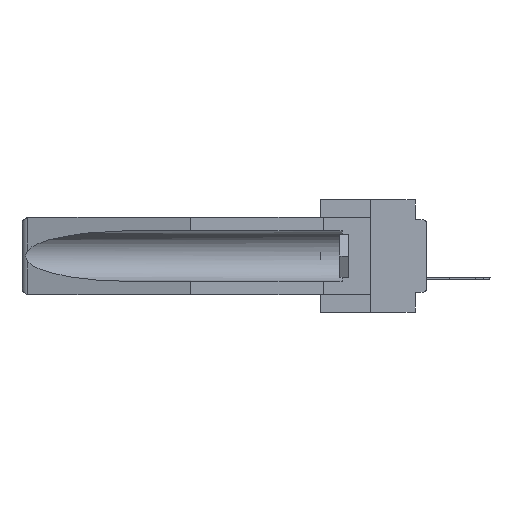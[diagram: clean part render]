
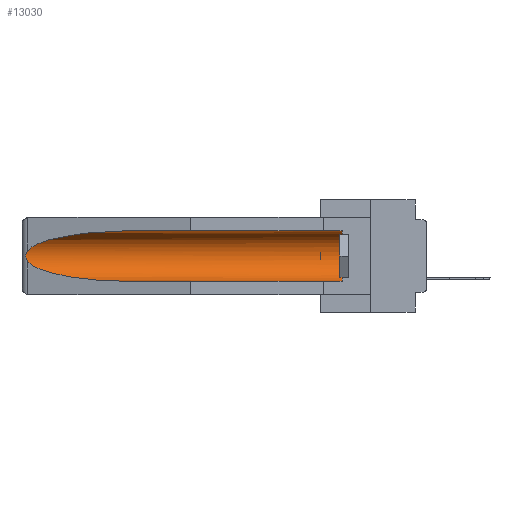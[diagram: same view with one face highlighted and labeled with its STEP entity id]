
A CAD part, left-side view. The second image highlights one B-rep face of the part: STEP entity #13030.
In plain terms, the highlighted cylindrical face has radius 2.857 mm (diameter 5.715 mm), a partial arc.
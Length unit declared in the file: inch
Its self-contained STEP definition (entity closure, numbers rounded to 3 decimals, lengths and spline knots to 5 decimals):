
#1356 = CARTESIAN_POINT ( 'NONE',  ( 0.26597, 1.5296, -0.19026 ) ) ;
#1966 = AXIS2_PLACEMENT_3D ( 'NONE', #36388, #32983, #39023 ) ;
#2346 = CARTESIAN_POINT ( 'NONE',  ( 0.26537, 1.52718, -0.19328 ) ) ;
#2478 = CARTESIAN_POINT ( 'NONE',  ( 0.155, 1.07973, -0.284 ) ) ;
#2673 = DIRECTION ( 'NONE',  ( 0., 1., 0. ) ) ;
#2771 = ORIENTED_EDGE ( 'NONE', *, *, #6622, .T. ) ;
#2885 = B_SPLINE_CURVE_WITH_KNOTS ( 'NONE', 3,
 ( #12368, #5298, #27321, #39610, #24892, #18644, #30938, #13312, #1356, #13907 ),
 .UNSPECIFIED., .F., .F.,
 ( 4, 2, 2, 2, 4 ),
 ( 0., 0.00029, 0.00058, 0.00087, 0.00117 ),
 .UNSPECIFIED. ) ;
#3277 = LINE ( 'NONE', #30534, #9221 ) ;
#4219 = VECTOR ( 'NONE', #39532, 39.37008 ) ;
#4569 = CIRCLE ( 'NONE', #1966, 0.1125 ) ;
#4816 = DIRECTION ( 'NONE',  ( 0., 0., 1. ) ) ;
#5298 = CARTESIAN_POINT ( 'NONE',  ( 0.26597, 1.52961, -0.15275 ) ) ;
#5886 = CARTESIAN_POINT ( 'NONE',  ( 0.26537, 1.52718, -0.14972 ) ) ;
#6622 = EDGE_CURVE ( 'NONE', #8143, #30828, #2885, .T. ) ;
#6766 = CARTESIAN_POINT ( 'NONE',  ( 0.26537, 1.52718, -0.14972 ) ) ;
#7658 = EDGE_CURVE ( 'NONE', #30828, #13727, #8458, .T. ) ;
#8143 = VERTEX_POINT ( 'NONE', #5886 ) ;
#8458 =( BOUNDED_CURVE ( )  B_SPLINE_CURVE ( 3, ( #2346, #13892, #14704, #26816 ),
 .UNSPECIFIED., .F., .F. ) 
 B_SPLINE_CURVE_WITH_KNOTS ( ( 4, 4 ),
 ( 0.1948, 1.5708 ),
 .UNSPECIFIED. ) 
 CURVE ( )  GEOMETRIC_REPRESENTATION_ITEM ( )  RATIONAL_B_SPLINE_CURVE ( ( 1., 0.848, 0.848, 1. ) ) 
 REPRESENTATION_ITEM ( '' )  );
#9221 = VECTOR ( 'NONE', #2673, 39.37008 ) ;
#9334 = EDGE_LOOP ( 'NONE', ( #15441, #2771, #26582, #38266, #13902, #19964 ) ) ;
#10158 = EDGE_CURVE ( 'NONE', #10968, #8143, #21922, .T. ) ;
#10476 = CYLINDRICAL_SURFACE ( 'NONE', #32827, 0.1125 ) ;
#10968 = VERTEX_POINT ( 'NONE', #15533 ) ;
#11083 = CARTESIAN_POINT ( 'NONE',  ( 0.155, -0.30754, -0.1715 ) ) ;
#12368 = CARTESIAN_POINT ( 'NONE',  ( 0.26537, 1.52718, -0.14972 ) ) ;
#13030 = ADVANCED_FACE ( 'NONE', ( #13712 ), #10476, .F. ) ;
#13312 = CARTESIAN_POINT ( 'NONE',  ( 0.26655, 1.53094, -0.18657 ) ) ;
#13712 = FACE_OUTER_BOUND ( 'NONE', #9334, .T. ) ;
#13727 = VERTEX_POINT ( 'NONE', #2478 ) ;
#13809 = CARTESIAN_POINT ( 'NONE',  ( 0.155, 0.126, -0.059 ) ) ;
#13892 = CARTESIAN_POINT ( 'NONE',  ( 0.25451, 1.48313, -0.24835 ) ) ;
#13902 = ORIENTED_EDGE ( 'NONE', *, *, #17924, .T. ) ;
#13907 = CARTESIAN_POINT ( 'NONE',  ( 0.26537, 1.52718, -0.19328 ) ) ;
#14704 = CARTESIAN_POINT ( 'NONE',  ( 0.21114, 1.30732, -0.284 ) ) ;
#15441 = ORIENTED_EDGE ( 'NONE', *, *, #10158, .T. ) ;
#15533 = CARTESIAN_POINT ( 'NONE',  ( 0.155, 1.07973, -0.059 ) ) ;
#17759 = CARTESIAN_POINT ( 'NONE',  ( 0.155, -0.30754, -0.284 ) ) ;
#17924 = EDGE_CURVE ( 'NONE', #27974, #25676, #4569, .T. ) ;
#18644 = CARTESIAN_POINT ( 'NONE',  ( 0.2675, 1.53308, -0.17534 ) ) ;
#18715 = CARTESIAN_POINT ( 'NONE',  ( 0.21114, 1.30732, -0.059 ) ) ;
#19964 = ORIENTED_EDGE ( 'NONE', *, *, #23916, .T. ) ;
#21922 =( BOUNDED_CURVE ( )  B_SPLINE_CURVE ( 3, ( #34418, #18715, #31002, #6766 ),
 .UNSPECIFIED., .F., .T. ) 
 B_SPLINE_CURVE_WITH_KNOTS ( ( 4, 4 ),
 ( 4.71239, 6.08839 ),
 .UNSPECIFIED. ) 
 CURVE ( )  GEOMETRIC_REPRESENTATION_ITEM ( )  RATIONAL_B_SPLINE_CURVE ( ( 1., 0.848, 0.848, 1. ) ) 
 REPRESENTATION_ITEM ( '' )  );
#22816 = DIRECTION ( 'NONE',  ( 0., 1., 0. ) ) ;
#23916 = EDGE_CURVE ( 'NONE', #25676, #10968, #3277, .T. ) ;
#24892 = CARTESIAN_POINT ( 'NONE',  ( 0.2675, 1.53308, -0.16763 ) ) ;
#25676 = VERTEX_POINT ( 'NONE', #13809 ) ;
#26582 = ORIENTED_EDGE ( 'NONE', *, *, #7658, .T. ) ;
#26816 = CARTESIAN_POINT ( 'NONE',  ( 0.155, 1.07973, -0.284 ) ) ;
#27321 = CARTESIAN_POINT ( 'NONE',  ( 0.26654, 1.53092, -0.15636 ) ) ;
#27974 = VERTEX_POINT ( 'NONE', #36399 ) ;
#30534 = CARTESIAN_POINT ( 'NONE',  ( 0.155, -0.30754, -0.059 ) ) ;
#30828 = VERTEX_POINT ( 'NONE', #38042 ) ;
#30938 = CARTESIAN_POINT ( 'NONE',  ( 0.2673, 1.53269, -0.17917 ) ) ;
#31002 = CARTESIAN_POINT ( 'NONE',  ( 0.25451, 1.48313, -0.09465 ) ) ;
#32827 = AXIS2_PLACEMENT_3D ( 'NONE', #11083, #22816, #4816 ) ;
#32983 = DIRECTION ( 'NONE',  ( 0., -1., 0. ) ) ;
#33095 = LINE ( 'NONE', #17759, #4219 ) ;
#34418 = CARTESIAN_POINT ( 'NONE',  ( 0.155, 1.07973, -0.059 ) ) ;
#36388 = CARTESIAN_POINT ( 'NONE',  ( 0.155, 0.126, -0.1715 ) ) ;
#36399 = CARTESIAN_POINT ( 'NONE',  ( 0.155, 0.126, -0.284 ) ) ;
#36586 = EDGE_CURVE ( 'NONE', #27974, #13727, #33095, .T. ) ;
#38042 = CARTESIAN_POINT ( 'NONE',  ( 0.26537, 1.52718, -0.19328 ) ) ;
#38266 = ORIENTED_EDGE ( 'NONE', *, *, #36586, .F. ) ;
#39023 = DIRECTION ( 'NONE',  ( 0., 0., 1. ) ) ;
#39532 = DIRECTION ( 'NONE',  ( 0., 1., 0. ) ) ;
#39610 = CARTESIAN_POINT ( 'NONE',  ( 0.2673, 1.5327, -0.16383 ) ) ;
